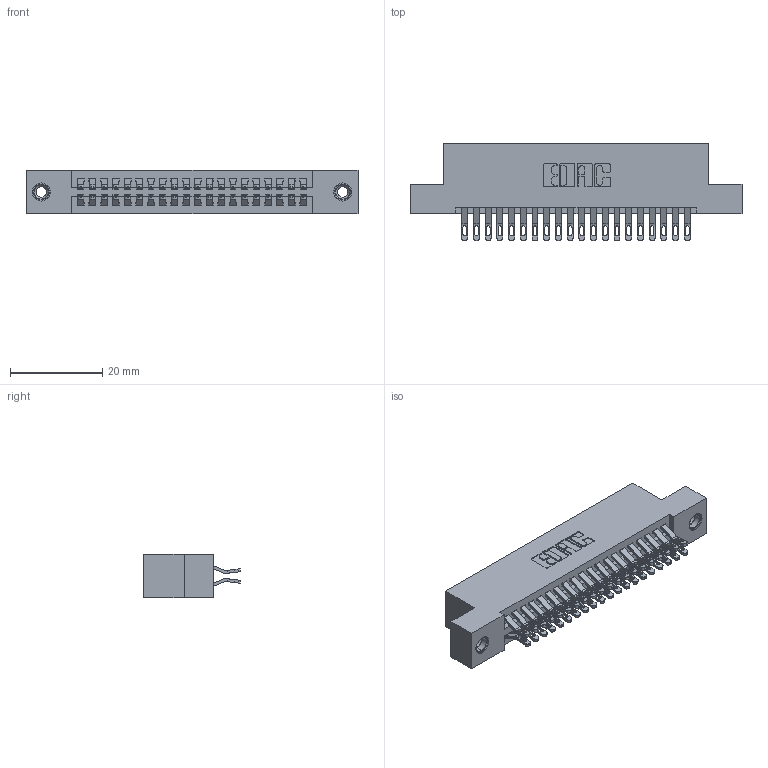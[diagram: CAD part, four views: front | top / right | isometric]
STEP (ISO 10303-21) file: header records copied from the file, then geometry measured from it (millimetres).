
FILE_DESCRIPTION (( 'STEP AP203' ), '1' );
FILE_NAME ('395-040-555-208.STEP', '2019-10-18T05:47:50', ( '' ), ( '' ), 'SwSTEP 2.0', 'SolidWorks 2016', '' );
FILE_SCHEMA (( 'CONFIG_CONTROL_DESIGN' ));
Length unit declared in the file: inch
Products named in the file (4): 345 Part_Flush Mounting Lugs - 0.156 Dia-TI; 345-292-001_555 Tail; 345-250-001_345-250-003-102; 395-040-555-208
Assembly tree (43 placements, depth 2):
  395-040-555-208
    345 Part_Flush Mounting Lugs - 0.156 Dia-TI
    345-292-001_555 Tail  x40
    345-250-001_345-250-003-102  x2
Bounding box: 72.01 x 21.13 x 9.4 mm (x, y, z)
Volume: 6900.3 mm3; surface area: 10190.7 mm2
Topology: 43 solids, 43 shells, 2426 faces, 7557 edges, 5030 vertices
Faces by surface type: plane 1352, cylinder 1058, cone 12, torus 4
Entity records: 20166 total; most frequent: CARTESIAN_POINT 3417, ORIENTED_EDGE 3314, DIRECTION 3035, EDGE_CURVE 1657, VECTOR 1405, LINE 1405, VERTEX_POINT 1100, AXIS2_PLACEMENT_3D 815
